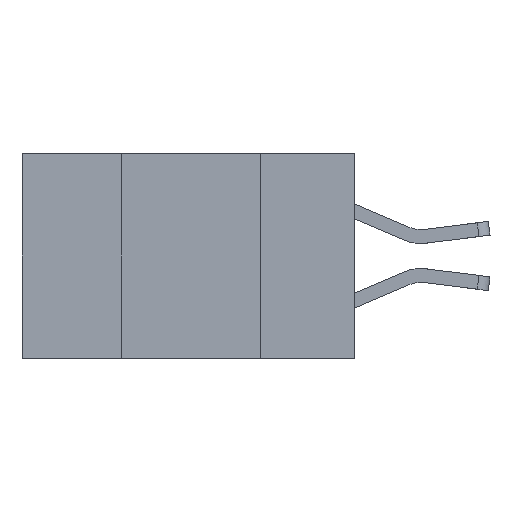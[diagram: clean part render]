
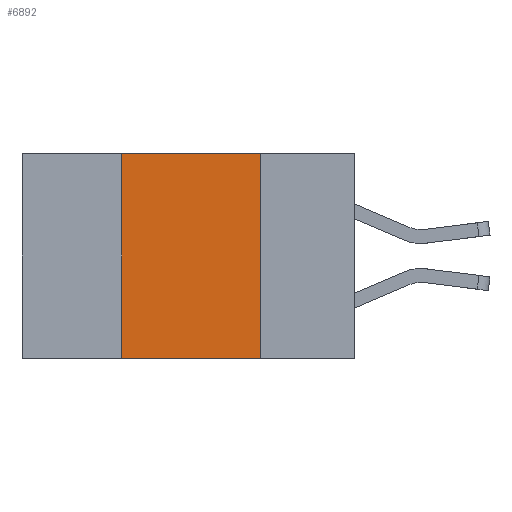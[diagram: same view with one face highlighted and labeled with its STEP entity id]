
A CAD part, left-side view. The second image highlights one B-rep face of the part: STEP entity #6892.
In plain terms, the highlighted planar face has unit normal (-1, 0, 0).
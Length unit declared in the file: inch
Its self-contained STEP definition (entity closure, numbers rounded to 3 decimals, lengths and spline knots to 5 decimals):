
#89 = EDGE_CURVE ( 'NONE', #5722, #7443, #5153, .T. ) ;
#203 = ORIENTED_EDGE ( 'NONE', *, *, #89, .F. ) ;
#1070 = EDGE_LOOP ( 'NONE', ( #10683, #203, #10371, #9186 ) ) ;
#1192 = DIRECTION ( 'NONE',  ( 0., 0., -1. ) ) ;
#1770 = CARTESIAN_POINT ( 'NONE',  ( 0., 0.42, 0. ) ) ;
#2049 = DIRECTION ( 'NONE',  ( 0., -1., 0. ) ) ;
#2702 = VECTOR ( 'NONE', #7322, 39.37008 ) ;
#3101 = CARTESIAN_POINT ( 'NONE',  ( 0., 0.6, 0. ) ) ;
#3590 = CARTESIAN_POINT ( 'NONE',  ( 0., 0.17, 0. ) ) ;
#3796 = DIRECTION ( 'NONE',  ( 0., 0., 1. ) ) ;
#4603 = LINE ( 'NONE', #7791, #10658 ) ;
#4909 = VECTOR ( 'NONE', #6465, 39.37008 ) ;
#5097 = LINE ( 'NONE', #10456, #2702 ) ;
#5153 = LINE ( 'NONE', #6229, #4909 ) ;
#5307 = EDGE_CURVE ( 'NONE', #7443, #10755, #5097, .T. ) ;
#5345 = EDGE_CURVE ( 'NONE', #10152, #5722, #9653, .T. ) ;
#5380 = EDGE_CURVE ( 'NONE', #10152, #10755, #4603, .T. ) ;
#5722 = VERTEX_POINT ( 'NONE', #1770 ) ;
#5732 = PLANE ( 'NONE',  #6521 ) ;
#5742 = CARTESIAN_POINT ( 'NONE',  ( 0., 0.17, -0.37 ) ) ;
#6229 = CARTESIAN_POINT ( 'NONE',  ( 0., 0.6, 0. ) ) ;
#6465 = DIRECTION ( 'NONE',  ( 0., -1., 0. ) ) ;
#6521 = AXIS2_PLACEMENT_3D ( 'NONE', #3101, #6549, #1192 ) ;
#6549 = DIRECTION ( 'NONE',  ( 1., 0., 0. ) ) ;
#6892 = ADVANCED_FACE ( 'NONE', ( #9525 ), #5732, .F. ) ;
#7322 = DIRECTION ( 'NONE',  ( 0., 0., -1. ) ) ;
#7443 = VERTEX_POINT ( 'NONE', #3590 ) ;
#7791 = CARTESIAN_POINT ( 'NONE',  ( 0., 0.6, -0.37 ) ) ;
#9186 = ORIENTED_EDGE ( 'NONE', *, *, #5380, .T. ) ;
#9417 = CARTESIAN_POINT ( 'NONE',  ( 0., 0.42, -0.37 ) ) ;
#9525 = FACE_OUTER_BOUND ( 'NONE', #1070, .T. ) ;
#9573 = CARTESIAN_POINT ( 'NONE',  ( 0., 0.42, 0. ) ) ;
#9653 = LINE ( 'NONE', #9573, #10881 ) ;
#10152 = VERTEX_POINT ( 'NONE', #9417 ) ;
#10371 = ORIENTED_EDGE ( 'NONE', *, *, #5345, .F. ) ;
#10456 = CARTESIAN_POINT ( 'NONE',  ( 0., 0.17, 0. ) ) ;
#10658 = VECTOR ( 'NONE', #2049, 39.37008 ) ;
#10683 = ORIENTED_EDGE ( 'NONE', *, *, #5307, .F. ) ;
#10755 = VERTEX_POINT ( 'NONE', #5742 ) ;
#10881 = VECTOR ( 'NONE', #3796, 39.37008 ) ;
